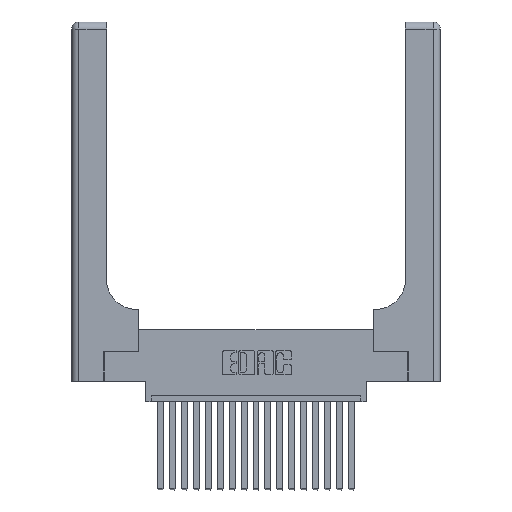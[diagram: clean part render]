
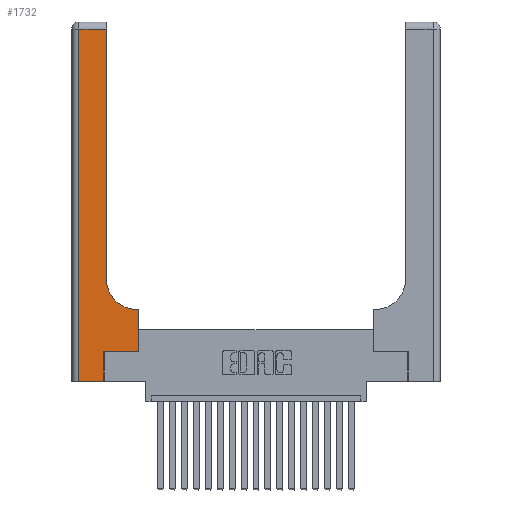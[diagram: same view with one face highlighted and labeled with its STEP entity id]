
A CAD part, top view. The second image highlights one B-rep face of the part: STEP entity #1732.
In plain terms, the highlighted planar face has unit normal (0, 0, 1).
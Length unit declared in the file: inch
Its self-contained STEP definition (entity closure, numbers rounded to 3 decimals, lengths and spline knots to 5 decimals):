
#327 = ORIENTED_EDGE ( 'NONE', *, *, #3638, .T. ) ;
#376 = ORIENTED_EDGE ( 'NONE', *, *, #20807, .T. ) ;
#729 = EDGE_LOOP ( 'NONE', ( #1325, #7853, #376, #8738, #12717, #7228, #2170, #2911, #327 ) ) ;
#878 = EDGE_CURVE ( 'NONE', #5578, #8097, #18591, .T. ) ;
#930 = PLANE ( 'NONE',  #3790 ) ;
#1325 = ORIENTED_EDGE ( 'NONE', *, *, #1500, .T. ) ;
#1500 = EDGE_CURVE ( 'NONE', #8352, #11748, #9038, .T. ) ;
#1631 = DIRECTION ( 'NONE',  ( -1., 0., 0. ) ) ;
#1732 = ADVANCED_FACE ( 'NONE', ( #6985 ), #930, .F. ) ;
#1765 = CARTESIAN_POINT ( 'NONE',  ( 0.2915, 0.85, 0.37 ) ) ;
#2041 = EDGE_CURVE ( 'NONE', #7989, #3471, #3609, .T. ) ;
#2170 = ORIENTED_EDGE ( 'NONE', *, *, #878, .T. ) ;
#2862 = CARTESIAN_POINT ( 'NONE',  ( 0.5585, 0.6, 0.37 ) ) ;
#2911 = ORIENTED_EDGE ( 'NONE', *, *, #10228, .T. ) ;
#3267 = CARTESIAN_POINT ( 'NONE',  ( 0.06, 0., 0.37 ) ) ;
#3471 = VERTEX_POINT ( 'NONE', #13796 ) ;
#3609 = LINE ( 'NONE', #14625, #20101 ) ;
#3638 = EDGE_CURVE ( 'NONE', #7714, #8352, #14174, .T. ) ;
#3790 = AXIS2_PLACEMENT_3D ( 'NONE', #6944, #4071, #13912 ) ;
#4071 = DIRECTION ( 'NONE',  ( 0., 0., -1. ) ) ;
#4110 = DIRECTION ( 'NONE',  ( -1., 0., 0. ) ) ;
#4522 = CARTESIAN_POINT ( 'NONE',  ( 0.2915, 3., 0.37 ) ) ;
#4735 = DIRECTION ( 'NONE',  ( 0., 1., 0. ) ) ;
#5442 = CARTESIAN_POINT ( 'NONE',  ( 0.2915, 2.94, 0.37 ) ) ;
#5578 = VERTEX_POINT ( 'NONE', #17401 ) ;
#5948 = LINE ( 'NONE', #8815, #9794 ) ;
#6730 = VERTEX_POINT ( 'NONE', #16941 ) ;
#6889 = DIRECTION ( 'NONE',  ( 1., 0., 0. ) ) ;
#6944 = CARTESIAN_POINT ( 'NONE',  ( 0., 3., 0.37 ) ) ;
#6985 = FACE_OUTER_BOUND ( 'NONE', #729, .T. ) ;
#7228 = ORIENTED_EDGE ( 'NONE', *, *, #8018, .T. ) ;
#7714 = VERTEX_POINT ( 'NONE', #19928 ) ;
#7853 = ORIENTED_EDGE ( 'NONE', *, *, #20189, .T. ) ;
#7989 = VERTEX_POINT ( 'NONE', #17515 ) ;
#8007 = CARTESIAN_POINT ( 'NONE',  ( 0., 2.94, 0.37 ) ) ;
#8009 = DIRECTION ( 'NONE',  ( 0., 1., 0. ) ) ;
#8018 = EDGE_CURVE ( 'NONE', #3471, #5578, #8607, .T. ) ;
#8097 = VERTEX_POINT ( 'NONE', #2862 ) ;
#8352 = VERTEX_POINT ( 'NONE', #1765 ) ;
#8412 = CARTESIAN_POINT ( 'NONE',  ( 0.06, 3., 0.37 ) ) ;
#8607 = LINE ( 'NONE', #17298, #19943 ) ;
#8738 = ORIENTED_EDGE ( 'NONE', *, *, #16936, .T. ) ;
#8815 = CARTESIAN_POINT ( 'NONE',  ( 0., 0., 0.37 ) ) ;
#9038 = LINE ( 'NONE', #4522, #15993 ) ;
#9794 = VECTOR ( 'NONE', #6889, 39.37008 ) ;
#10228 = EDGE_CURVE ( 'NONE', #8097, #7714, #13897, .T. ) ;
#10761 = DIRECTION ( 'NONE',  ( 1., 0., 0. ) ) ;
#11294 = CARTESIAN_POINT ( 'NONE',  ( 0.5585, 0.25, 0.37 ) ) ;
#11748 = VERTEX_POINT ( 'NONE', #5442 ) ;
#12717 = ORIENTED_EDGE ( 'NONE', *, *, #2041, .T. ) ;
#13304 = DIRECTION ( 'NONE',  ( 0., -1., 0. ) ) ;
#13796 = CARTESIAN_POINT ( 'NONE',  ( 0.269, 0.25, 0.37 ) ) ;
#13897 = LINE ( 'NONE', #13960, #14150 ) ;
#13912 = DIRECTION ( 'NONE',  ( -1., 0., 0. ) ) ;
#13918 = CARTESIAN_POINT ( 'NONE',  ( 0.5415, 0.85, 0.37 ) ) ;
#13960 = CARTESIAN_POINT ( 'NONE',  ( 0.2915, 0.6, 0.37 ) ) ;
#14058 = VERTEX_POINT ( 'NONE', #3267 ) ;
#14150 = VECTOR ( 'NONE', #4110, 39.37008 ) ;
#14174 = CIRCLE ( 'NONE', #16087, 0.25 ) ;
#14625 = CARTESIAN_POINT ( 'NONE',  ( 0.269, 0., 0.37 ) ) ;
#15982 = DIRECTION ( 'NONE',  ( 0., 1., 0. ) ) ;
#15993 = VECTOR ( 'NONE', #4735, 39.37008 ) ;
#16087 = AXIS2_PLACEMENT_3D ( 'NONE', #13918, #19032, #19178 ) ;
#16936 = EDGE_CURVE ( 'NONE', #14058, #7989, #5948, .T. ) ;
#16941 = CARTESIAN_POINT ( 'NONE',  ( 0.06, 2.94, 0.37 ) ) ;
#17289 = VECTOR ( 'NONE', #15982, 39.37008 ) ;
#17298 = CARTESIAN_POINT ( 'NONE',  ( 0.269, 0.25, 0.37 ) ) ;
#17401 = CARTESIAN_POINT ( 'NONE',  ( 0.5585, 0.25, 0.37 ) ) ;
#17515 = CARTESIAN_POINT ( 'NONE',  ( 0.269, 0., 0.37 ) ) ;
#18591 = LINE ( 'NONE', #11294, #17289 ) ;
#19032 = DIRECTION ( 'NONE',  ( 0., 0., -1. ) ) ;
#19178 = DIRECTION ( 'NONE',  ( 1., 0., 0. ) ) ;
#19186 = VECTOR ( 'NONE', #13304, 39.37008 ) ;
#19494 = VECTOR ( 'NONE', #1631, 39.37008 ) ;
#19928 = CARTESIAN_POINT ( 'NONE',  ( 0.5415, 0.6, 0.37 ) ) ;
#19943 = VECTOR ( 'NONE', #10761, 39.37008 ) ;
#20009 = LINE ( 'NONE', #8007, #19494 ) ;
#20101 = VECTOR ( 'NONE', #8009, 39.37008 ) ;
#20189 = EDGE_CURVE ( 'NONE', #11748, #6730, #20009, .T. ) ;
#20807 = EDGE_CURVE ( 'NONE', #6730, #14058, #21252, .T. ) ;
#21252 = LINE ( 'NONE', #8412, #19186 ) ;
